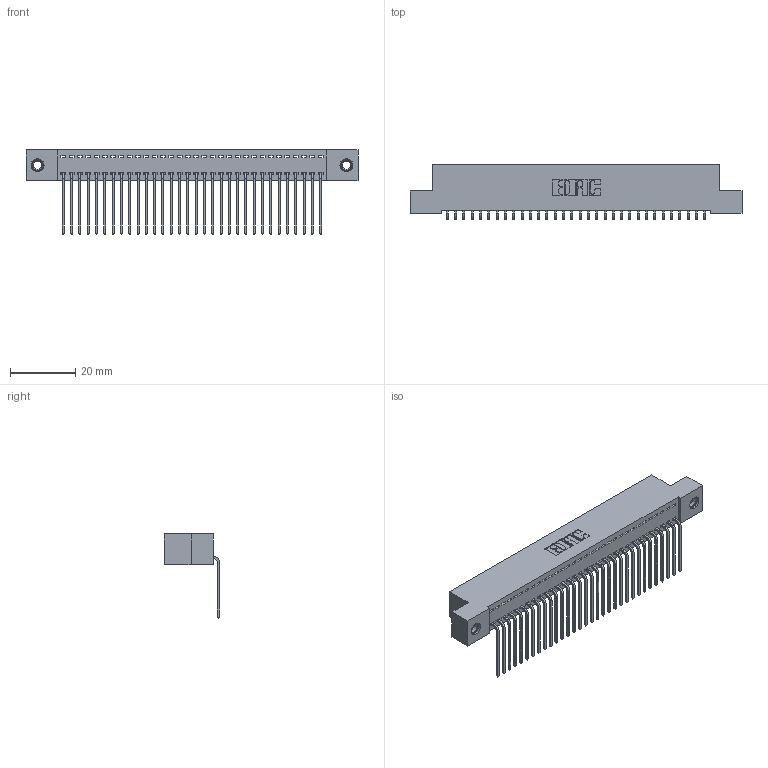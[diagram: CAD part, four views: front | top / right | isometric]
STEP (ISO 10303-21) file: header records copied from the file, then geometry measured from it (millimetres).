
FILE_DESCRIPTION (( 'STEP AP203' ), '1' );
FILE_NAME ('342-032-559-107.STEP', '2019-10-02T11:25:57', ( '' ), ( '' ), 'SwSTEP 2.0', 'SolidWorks 2016', '' );
FILE_SCHEMA (( 'CONFIG_CONTROL_DESIGN' ));
Length unit declared in the file: inch
Products named in the file (4): 345-250-001_345-250-005-103; 342-032-559-107; 342 Part_TI; 345-292-001_558 559 Tail - 1
Assembly tree (35 placements, depth 2):
  342-032-559-107
    342 Part_TI
    345-292-001_558 559 Tail - 1  x32
    345-250-001_345-250-005-103  x2
Bounding box: 101.6 x 16.83 x 25.78 mm (x, y, z)
Volume: 8965.4 mm3; surface area: 13616.3 mm2
Topology: 35 solids, 35 shells, 2090 faces, 6259 edges, 4122 vertices
Faces by surface type: plane 1506, cylinder 568, cone 12, torus 4
Entity records: 21994 total; most frequent: CARTESIAN_POINT 3777, ORIENTED_EDGE 3738, DIRECTION 3239, EDGE_CURVE 1869, LINE 1721, VECTOR 1721, VERTEX_POINT 1240, AXIS2_PLACEMENT_3D 759
